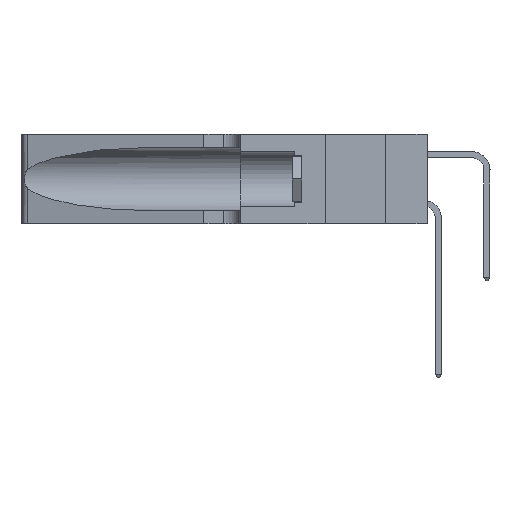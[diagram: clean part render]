
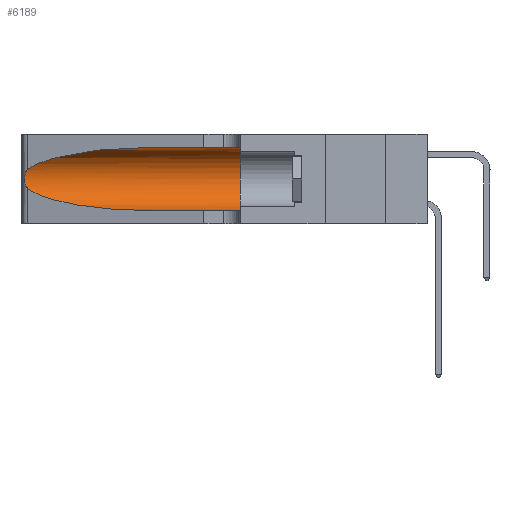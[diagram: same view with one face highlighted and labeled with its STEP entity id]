
A CAD part, left-side view. The second image highlights one B-rep face of the part: STEP entity #6189.
In plain terms, the highlighted cylindrical face has radius 3.308 mm (diameter 6.617 mm), a partial arc.
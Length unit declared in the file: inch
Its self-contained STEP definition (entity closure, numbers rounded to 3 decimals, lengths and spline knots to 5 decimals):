
#51 = EDGE_CURVE ( 'NONE', #33549, #22483, #13044, .T. ) ;
#120 = DIRECTION ( 'NONE',  ( 0., 0., 1. ) ) ;
#389 = CARTESIAN_POINT ( 'NONE',  ( 0.1305, 0.35, 0.31525 ) ) ;
#815 = CARTESIAN_POINT ( 'NONE',  ( 0.18966, 0.96281, 0.31525 ) ) ;
#1123 = CARTESIAN_POINT ( 'NONE',  ( 0.25789, 1.23486, 0.15765 ) ) ;
#1657 =( BOUNDED_CURVE ( )  B_SPLINE_CURVE ( 3, ( #17515, #24873, #11812, #14733 ),
 .UNSPECIFIED., .F., .F. ) 
 B_SPLINE_CURVE_WITH_KNOTS ( ( 4, 4 ),
 ( 3.44316, 4.71239 ),
 .UNSPECIFIED. ) 
 CURVE ( )  GEOMETRIC_REPRESENTATION_ITEM ( )  RATIONAL_B_SPLINE_CURVE ( ( 1., 0.87, 0.87, 1. ) ) 
 REPRESENTATION_ITEM ( '' )  );
#1750 = CARTESIAN_POINT ( 'NONE',  ( 0.25487, 1.22718, 0.22369 ) ) ;
#2003 = CARTESIAN_POINT ( 'NONE',  ( 0.1305, 1.61858, 0.05475 ) ) ;
#2396 = EDGE_CURVE ( 'NONE', #18879, #22483, #23265, .T. ) ;
#2871 = ORIENTED_EDGE ( 'NONE', *, *, #21535, .F. ) ;
#3708 = CARTESIAN_POINT ( 'NONE',  ( 0.2373, 1.15595, 0.28018 ) ) ;
#3786 = CARTESIAN_POINT ( 'NONE',  ( 0.25555, 1.22993, 0.14849 ) ) ;
#4389 = CARTESIAN_POINT ( 'NONE',  ( 0.26018, 1.23835, 0.19895 ) ) ;
#5036 = CARTESIAN_POINT ( 'NONE',  ( 0.1305, 1.61858, 0.185 ) ) ;
#5650 = B_SPLINE_CURVE_WITH_KNOTS ( 'NONE', 3,
 ( #1750, #15045, #14084, #11524, #32660, #4389, #28264, #8871, #20373, #33008, #1123, #25577, #3786, #6200 ),
 .UNSPECIFIED., .F., .F.,
 ( 4, 2, 2, 2, 2, 2, 4 ),
 ( 0., 0.00027, 0.00053, 0.00107, 0.0016, 0.00187, 0.00214 ),
 .UNSPECIFIED. ) ;
#5988 = CARTESIAN_POINT ( 'NONE',  ( 0.25487, 1.22718, 0.22369 ) ) ;
#6189 = ADVANCED_FACE ( 'NONE', ( #31147 ), #31949, .F. ) ;
#6200 = CARTESIAN_POINT ( 'NONE',  ( 0.25487, 1.22718, 0.14631 ) ) ;
#6915 = CARTESIAN_POINT ( 'NONE',  ( 0.1305, 0.35, 0.05475 ) ) ;
#7158 = ORIENTED_EDGE ( 'NONE', *, *, #51, .F. ) ;
#8871 = CARTESIAN_POINT ( 'NONE',  ( 0.26075, 1.23896, 0.178 ) ) ;
#10036 = CARTESIAN_POINT ( 'NONE',  ( 0.1305, 0.72297, 0.05475 ) ) ;
#11524 = CARTESIAN_POINT ( 'NONE',  ( 0.25787, 1.23484, 0.2124 ) ) ;
#11812 = CARTESIAN_POINT ( 'NONE',  ( 0.18966, 0.96281, 0.05475 ) ) ;
#12182 = CARTESIAN_POINT ( 'NONE',  ( 0.25487, 1.22718, 0.14631 ) ) ;
#13044 = CIRCLE ( 'NONE', #14240, 0.13025 ) ;
#13314 = EDGE_CURVE ( 'NONE', #24544, #30622, #5650, .T. ) ;
#13480 = VECTOR ( 'NONE', #29271, 39.37008 ) ;
#14084 = CARTESIAN_POINT ( 'NONE',  ( 0.25639, 1.23184, 0.21858 ) ) ;
#14240 = AXIS2_PLACEMENT_3D ( 'NONE', #14765, #20086, #120 ) ;
#14733 = CARTESIAN_POINT ( 'NONE',  ( 0.1305, 0.72297, 0.05475 ) ) ;
#14765 = CARTESIAN_POINT ( 'NONE',  ( 0.1305, 0.35, 0.185 ) ) ;
#15045 = CARTESIAN_POINT ( 'NONE',  ( 0.25555, 1.22994, 0.2215 ) ) ;
#15701 = AXIS2_PLACEMENT_3D ( 'NONE', #5036, #23560, #25798 ) ;
#16440 = ORIENTED_EDGE ( 'NONE', *, *, #26795, .T. ) ;
#16473 =( BOUNDED_CURVE ( )  B_SPLINE_CURVE ( 3, ( #25115, #815, #3708, #19308 ),
 .UNSPECIFIED., .F., .F. ) 
 B_SPLINE_CURVE_WITH_KNOTS ( ( 4, 4 ),
 ( 1.5708, 2.84003 ),
 .UNSPECIFIED. ) 
 CURVE ( )  GEOMETRIC_REPRESENTATION_ITEM ( )  RATIONAL_B_SPLINE_CURVE ( ( 1., 0.87, 0.87, 1. ) ) 
 REPRESENTATION_ITEM ( '' )  );
#17515 = CARTESIAN_POINT ( 'NONE',  ( 0.25487, 1.22718, 0.14631 ) ) ;
#18263 = ORIENTED_EDGE ( 'NONE', *, *, #2396, .T. ) ;
#18879 = VERTEX_POINT ( 'NONE', #10036 ) ;
#19308 = CARTESIAN_POINT ( 'NONE',  ( 0.25487, 1.22718, 0.22369 ) ) ;
#19543 = EDGE_CURVE ( 'NONE', #21521, #24544, #16473, .T. ) ;
#20086 = DIRECTION ( 'NONE',  ( 0., 1., 0. ) ) ;
#20195 = CARTESIAN_POINT ( 'NONE',  ( 0.1305, 0.72297, 0.31525 ) ) ;
#20373 = CARTESIAN_POINT ( 'NONE',  ( 0.26017, 1.23833, 0.17102 ) ) ;
#21521 = VERTEX_POINT ( 'NONE', #20195 ) ;
#21535 = EDGE_CURVE ( 'NONE', #21521, #33549, #23026, .T. ) ;
#22172 = CARTESIAN_POINT ( 'NONE',  ( 0.1305, 1.61858, 0.31525 ) ) ;
#22438 = ORIENTED_EDGE ( 'NONE', *, *, #19543, .T. ) ;
#22483 = VERTEX_POINT ( 'NONE', #6915 ) ;
#23026 = LINE ( 'NONE', #22172, #13480 ) ;
#23265 = LINE ( 'NONE', #2003, #26581 ) ;
#23560 = DIRECTION ( 'NONE',  ( 0., -1., 0. ) ) ;
#24544 = VERTEX_POINT ( 'NONE', #5988 ) ;
#24873 = CARTESIAN_POINT ( 'NONE',  ( 0.2373, 1.15595, 0.08982 ) ) ;
#25115 = CARTESIAN_POINT ( 'NONE',  ( 0.1305, 0.72297, 0.31525 ) ) ;
#25577 = CARTESIAN_POINT ( 'NONE',  ( 0.25639, 1.23186, 0.15144 ) ) ;
#25798 = DIRECTION ( 'NONE',  ( 0., 0., -1. ) ) ;
#25898 = EDGE_LOOP ( 'NONE', ( #22438, #34292, #16440, #18263, #7158, #2871 ) ) ;
#26581 = VECTOR ( 'NONE', #31335, 39.37008 ) ;
#26795 = EDGE_CURVE ( 'NONE', #30622, #18879, #1657, .T. ) ;
#28264 = CARTESIAN_POINT ( 'NONE',  ( 0.26075, 1.23896, 0.19203 ) ) ;
#29271 = DIRECTION ( 'NONE',  ( 0., -1., 0. ) ) ;
#30622 = VERTEX_POINT ( 'NONE', #12182 ) ;
#31147 = FACE_OUTER_BOUND ( 'NONE', #25898, .T. ) ;
#31335 = DIRECTION ( 'NONE',  ( 0., -1., 0. ) ) ;
#31949 = CYLINDRICAL_SURFACE ( 'NONE', #15701, 0.13025 ) ;
#32660 = CARTESIAN_POINT ( 'NONE',  ( 0.25854, 1.2359, 0.20912 ) ) ;
#33008 = CARTESIAN_POINT ( 'NONE',  ( 0.25856, 1.23593, 0.16098 ) ) ;
#33549 = VERTEX_POINT ( 'NONE', #389 ) ;
#34292 = ORIENTED_EDGE ( 'NONE', *, *, #13314, .T. ) ;
